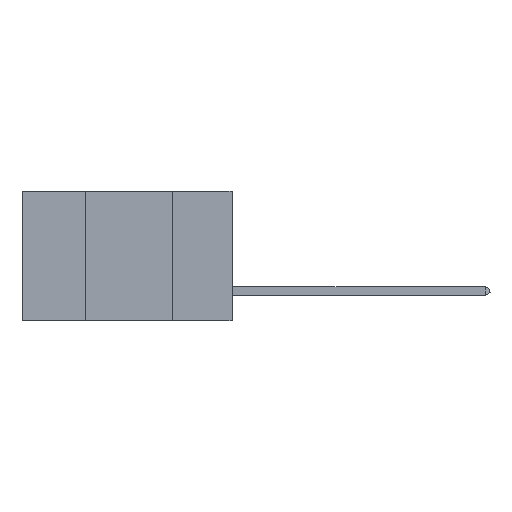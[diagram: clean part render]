
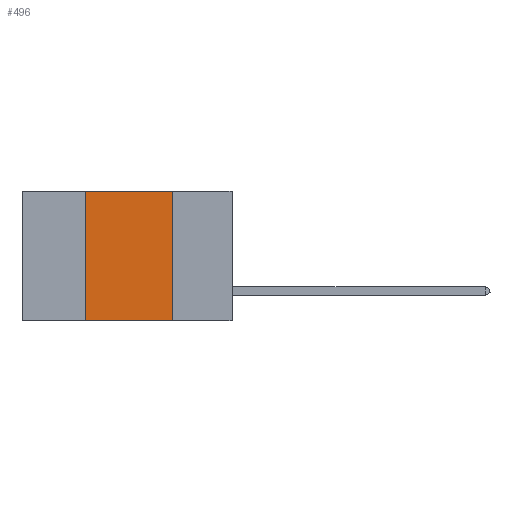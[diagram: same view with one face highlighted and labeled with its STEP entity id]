
A CAD part, left-side view. The second image highlights one B-rep face of the part: STEP entity #496.
In plain terms, the highlighted planar face has unit normal (-1, 0, 0).
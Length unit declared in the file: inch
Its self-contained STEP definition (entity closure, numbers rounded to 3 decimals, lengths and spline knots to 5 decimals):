
#126 = CARTESIAN_POINT ( 'NONE',  ( 0., 0.42, 0. ) ) ;
#496 = ADVANCED_FACE ( 'NONE', ( #12586 ), #8943, .F. ) ;
#575 = VERTEX_POINT ( 'NONE', #6692 ) ;
#1133 = VECTOR ( 'NONE', #7224, 39.37008 ) ;
#1275 = VECTOR ( 'NONE', #15350, 39.37008 ) ;
#1630 = CARTESIAN_POINT ( 'NONE',  ( 0., 0.17, -0.37 ) ) ;
#2451 = CARTESIAN_POINT ( 'NONE',  ( 0., 0.6, 0. ) ) ;
#4012 = ORIENTED_EDGE ( 'NONE', *, *, #6702, .F. ) ;
#4268 = LINE ( 'NONE', #10150, #4854 ) ;
#4305 = LINE ( 'NONE', #2451, #1275 ) ;
#4854 = VECTOR ( 'NONE', #9002, 39.37008 ) ;
#5621 = EDGE_LOOP ( 'NONE', ( #5719, #14978, #4012, #15122 ) ) ;
#5719 = ORIENTED_EDGE ( 'NONE', *, *, #7776, .F. ) ;
#6093 = VERTEX_POINT ( 'NONE', #1630 ) ;
#6321 = CARTESIAN_POINT ( 'NONE',  ( 0., 0.42, -0.37 ) ) ;
#6388 = DIRECTION ( 'NONE',  ( 0., 0., -1. ) ) ;
#6692 = CARTESIAN_POINT ( 'NONE',  ( 0., 0.42, 0. ) ) ;
#6702 = EDGE_CURVE ( 'NONE', #8295, #575, #14289, .T. ) ;
#7224 = DIRECTION ( 'NONE',  ( 0., 0., -1. ) ) ;
#7776 = EDGE_CURVE ( 'NONE', #16499, #6093, #12047, .T. ) ;
#8232 = AXIS2_PLACEMENT_3D ( 'NONE', #12788, #16468, #6388 ) ;
#8295 = VERTEX_POINT ( 'NONE', #6321 ) ;
#8943 = PLANE ( 'NONE',  #8232 ) ;
#9002 = DIRECTION ( 'NONE',  ( 0., -1., 0. ) ) ;
#9304 = EDGE_CURVE ( 'NONE', #575, #16499, #4305, .T. ) ;
#10150 = CARTESIAN_POINT ( 'NONE',  ( 0., 0.6, -0.37 ) ) ;
#10519 = DIRECTION ( 'NONE',  ( 0., 0., 1. ) ) ;
#10854 = VECTOR ( 'NONE', #10519, 39.37008 ) ;
#11975 = CARTESIAN_POINT ( 'NONE',  ( 0., 0.17, 0. ) ) ;
#12047 = LINE ( 'NONE', #14936, #1133 ) ;
#12586 = FACE_OUTER_BOUND ( 'NONE', #5621, .T. ) ;
#12788 = CARTESIAN_POINT ( 'NONE',  ( 0., 0.6, 0. ) ) ;
#14289 = LINE ( 'NONE', #126, #10854 ) ;
#14522 = EDGE_CURVE ( 'NONE', #8295, #6093, #4268, .T. ) ;
#14936 = CARTESIAN_POINT ( 'NONE',  ( 0., 0.17, 0. ) ) ;
#14978 = ORIENTED_EDGE ( 'NONE', *, *, #9304, .F. ) ;
#15122 = ORIENTED_EDGE ( 'NONE', *, *, #14522, .T. ) ;
#15350 = DIRECTION ( 'NONE',  ( 0., -1., 0. ) ) ;
#16468 = DIRECTION ( 'NONE',  ( 1., 0., 0. ) ) ;
#16499 = VERTEX_POINT ( 'NONE', #11975 ) ;
